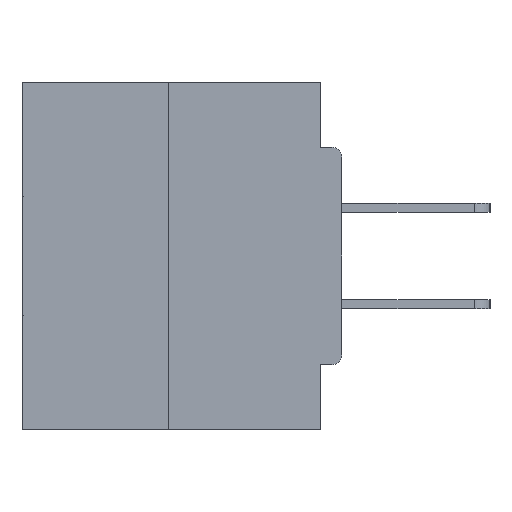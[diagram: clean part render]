
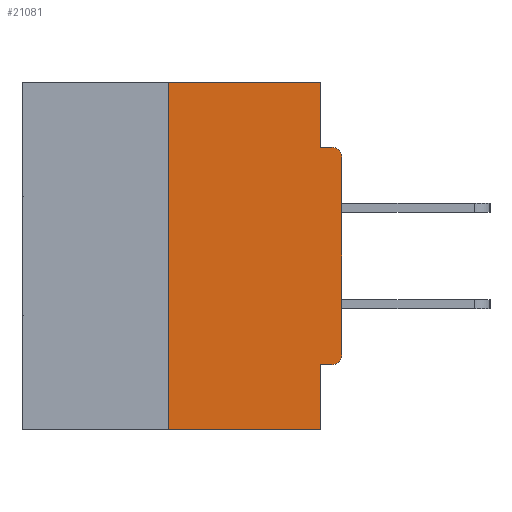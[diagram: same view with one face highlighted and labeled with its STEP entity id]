
A CAD part, left-side view. The second image highlights one B-rep face of the part: STEP entity #21081.
In plain terms, the highlighted planar face has unit normal (-1, 0, 0).
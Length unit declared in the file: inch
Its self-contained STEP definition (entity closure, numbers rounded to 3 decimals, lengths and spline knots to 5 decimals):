
#196 = CARTESIAN_POINT ( 'NONE',  ( 0., 0.46, 0. ) ) ;
#249 = CARTESIAN_POINT ( 'NONE',  ( 0., 0.031, -0.5 ) ) ;
#356 = VERTEX_POINT ( 'NONE', #12807 ) ;
#566 = CARTESIAN_POINT ( 'NONE',  ( 0., 0.25, 0. ) ) ;
#821 = DIRECTION ( 'NONE',  ( 0., 0., -1. ) ) ;
#3477 = CARTESIAN_POINT ( 'NONE',  ( 0., 0.031, -0.5 ) ) ;
#3502 = EDGE_CURVE ( 'NONE', #7270, #4870, #21834, .T. ) ;
#3753 = CARTESIAN_POINT ( 'NONE',  ( 0., 0., -0.4065 ) ) ;
#4452 = CARTESIAN_POINT ( 'NONE',  ( 0., 0.015, -0.4065 ) ) ;
#4870 = VERTEX_POINT ( 'NONE', #33533 ) ;
#5094 = CARTESIAN_POINT ( 'NONE',  ( 0., 0., -0.3915 ) ) ;
#5177 = DIRECTION ( 'NONE',  ( 0., 0., -1. ) ) ;
#5182 = CARTESIAN_POINT ( 'NONE',  ( 0., 0.031, -0.4065 ) ) ;
#5438 = ORIENTED_EDGE ( 'NONE', *, *, #28324, .F. ) ;
#5974 = EDGE_CURVE ( 'NONE', #24174, #356, #12096, .T. ) ;
#6024 = DIRECTION ( 'NONE',  ( 0., -1., 0. ) ) ;
#6038 = ORIENTED_EDGE ( 'NONE', *, *, #36935, .F. ) ;
#6276 = DIRECTION ( 'NONE',  ( 0., 0., -1. ) ) ;
#6759 = VECTOR ( 'NONE', #22749, 39.37008 ) ;
#7270 = VERTEX_POINT ( 'NONE', #36701 ) ;
#7553 = VERTEX_POINT ( 'NONE', #3477 ) ;
#8176 = ORIENTED_EDGE ( 'NONE', *, *, #33052, .F. ) ;
#8680 = CIRCLE ( 'NONE', #19949, 0.015 ) ;
#9414 = CARTESIAN_POINT ( 'NONE',  ( 0., 0.015, -0.1085 ) ) ;
#10385 = CARTESIAN_POINT ( 'NONE',  ( 0., 0.25, -0.5 ) ) ;
#11114 = CARTESIAN_POINT ( 'NONE',  ( 0., 0.015, -0.3915 ) ) ;
#11358 = ORIENTED_EDGE ( 'NONE', *, *, #15202, .T. ) ;
#11718 = CARTESIAN_POINT ( 'NONE',  ( 0., 0.46, 0. ) ) ;
#12096 = LINE ( 'NONE', #196, #33517 ) ;
#12130 = AXIS2_PLACEMENT_3D ( 'NONE', #9414, #29507, #15008 ) ;
#12807 = CARTESIAN_POINT ( 'NONE',  ( 0., 0.031, 0. ) ) ;
#13376 = VECTOR ( 'NONE', #25067, 39.37008 ) ;
#13566 = EDGE_CURVE ( 'NONE', #19372, #14663, #8680, .T. ) ;
#14663 = VERTEX_POINT ( 'NONE', #5094 ) ;
#14799 = LINE ( 'NONE', #30382, #13376 ) ;
#15008 = DIRECTION ( 'NONE',  ( 0., 0., -1. ) ) ;
#15202 = EDGE_CURVE ( 'NONE', #14663, #7270, #23211, .T. ) ;
#19012 = LINE ( 'NONE', #37639, #6759 ) ;
#19372 = VERTEX_POINT ( 'NONE', #4452 ) ;
#19753 = VECTOR ( 'NONE', #32522, 39.37008 ) ;
#19802 = EDGE_LOOP ( 'NONE', ( #35896, #6038, #36961, #36814, #8176, #29664, #11358, #32438, #5438, #35631 ) ) ;
#19949 = AXIS2_PLACEMENT_3D ( 'NONE', #11114, #34313, #5177 ) ;
#20676 = LINE ( 'NONE', #249, #19753 ) ;
#20874 = PLANE ( 'NONE',  #21480 ) ;
#21081 = ADVANCED_FACE ( 'NONE', ( #22739 ), #20874, .F. ) ;
#21157 = EDGE_CURVE ( 'NONE', #356, #33248, #27737, .T. ) ;
#21480 = AXIS2_PLACEMENT_3D ( 'NONE', #11718, #29284, #6276 ) ;
#21824 = DIRECTION ( 'NONE',  ( 0., 0., 1. ) ) ;
#21834 = CIRCLE ( 'NONE', #12130, 0.015 ) ;
#22323 = VECTOR ( 'NONE', #32879, 39.37008 ) ;
#22739 = FACE_OUTER_BOUND ( 'NONE', #19802, .T. ) ;
#22749 = DIRECTION ( 'NONE',  ( 0., -1., 0. ) ) ;
#22781 = LINE ( 'NONE', #3753, #22323 ) ;
#23211 = LINE ( 'NONE', #36339, #31821 ) ;
#23950 = CARTESIAN_POINT ( 'NONE',  ( 0., 0.031, 0. ) ) ;
#24174 = VERTEX_POINT ( 'NONE', #566 ) ;
#24662 = CARTESIAN_POINT ( 'NONE',  ( 0., 0., -0.0935 ) ) ;
#25067 = DIRECTION ( 'NONE',  ( 0., 0., 1. ) ) ;
#27737 = LINE ( 'NONE', #23950, #33670 ) ;
#28208 = VERTEX_POINT ( 'NONE', #10385 ) ;
#28324 = EDGE_CURVE ( 'NONE', #33248, #4870, #37100, .T. ) ;
#28640 = EDGE_CURVE ( 'NONE', #35921, #7553, #20676, .T. ) ;
#29284 = DIRECTION ( 'NONE',  ( 1., 0., 0. ) ) ;
#29360 = VECTOR ( 'NONE', #33451, 39.37008 ) ;
#29507 = DIRECTION ( 'NONE',  ( -1., 0., 0. ) ) ;
#29664 = ORIENTED_EDGE ( 'NONE', *, *, #13566, .T. ) ;
#30382 = CARTESIAN_POINT ( 'NONE',  ( 0., 0.25, 0. ) ) ;
#31688 = EDGE_CURVE ( 'NONE', #28208, #7553, #19012, .T. ) ;
#31821 = VECTOR ( 'NONE', #21824, 39.37008 ) ;
#32438 = ORIENTED_EDGE ( 'NONE', *, *, #3502, .T. ) ;
#32522 = DIRECTION ( 'NONE',  ( 0., 0., -1. ) ) ;
#32879 = DIRECTION ( 'NONE',  ( 0., 1., 0. ) ) ;
#33052 = EDGE_CURVE ( 'NONE', #19372, #35921, #22781, .T. ) ;
#33248 = VERTEX_POINT ( 'NONE', #34022 ) ;
#33451 = DIRECTION ( 'NONE',  ( 0., -1., 0. ) ) ;
#33517 = VECTOR ( 'NONE', #6024, 39.37008 ) ;
#33533 = CARTESIAN_POINT ( 'NONE',  ( 0., 0.015, -0.0935 ) ) ;
#33670 = VECTOR ( 'NONE', #821, 39.37008 ) ;
#34022 = CARTESIAN_POINT ( 'NONE',  ( 0., 0.031, -0.0935 ) ) ;
#34313 = DIRECTION ( 'NONE',  ( -1., 0., 0. ) ) ;
#35631 = ORIENTED_EDGE ( 'NONE', *, *, #21157, .F. ) ;
#35896 = ORIENTED_EDGE ( 'NONE', *, *, #5974, .F. ) ;
#35921 = VERTEX_POINT ( 'NONE', #5182 ) ;
#36339 = CARTESIAN_POINT ( 'NONE',  ( 0., 0., 0. ) ) ;
#36701 = CARTESIAN_POINT ( 'NONE',  ( 0., 0., -0.1085 ) ) ;
#36814 = ORIENTED_EDGE ( 'NONE', *, *, #28640, .F. ) ;
#36935 = EDGE_CURVE ( 'NONE', #28208, #24174, #14799, .T. ) ;
#36961 = ORIENTED_EDGE ( 'NONE', *, *, #31688, .T. ) ;
#37100 = LINE ( 'NONE', #24662, #29360 ) ;
#37639 = CARTESIAN_POINT ( 'NONE',  ( 0., 0.46, -0.5 ) ) ;
